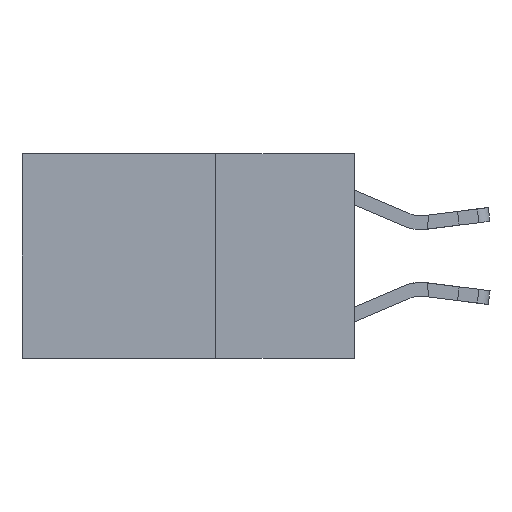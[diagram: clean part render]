
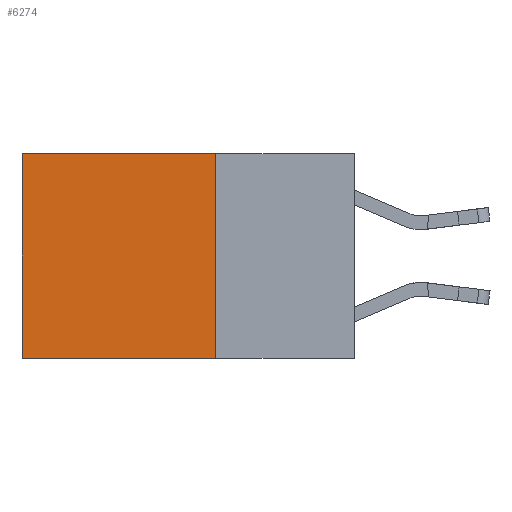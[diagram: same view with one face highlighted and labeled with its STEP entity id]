
A CAD part, left-side view. The second image highlights one B-rep face of the part: STEP entity #6274.
In plain terms, the highlighted planar face has unit normal (-1, 0, 0).
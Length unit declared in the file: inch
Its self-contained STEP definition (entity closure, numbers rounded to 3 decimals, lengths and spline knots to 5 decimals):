
#632 = DIRECTION ( 'NONE',  ( 0., 0., -1. ) ) ;
#649 = DIRECTION ( 'NONE',  ( 0., 1., 0. ) ) ;
#1404 = VECTOR ( 'NONE', #632, 39.37008 ) ;
#1470 = ORIENTED_EDGE ( 'NONE', *, *, #12815, .T. ) ;
#3358 = VERTEX_POINT ( 'NONE', #3982 ) ;
#3628 = LINE ( 'NONE', #10397, #16298 ) ;
#3683 = VECTOR ( 'NONE', #4352, 39.37008 ) ;
#3967 = DIRECTION ( 'NONE',  ( 0., 0., -1. ) ) ;
#3982 = CARTESIAN_POINT ( 'NONE',  ( 0.2625, 0.6, 0. ) ) ;
#4352 = DIRECTION ( 'NONE',  ( 0., 0., -1. ) ) ;
#4945 = LINE ( 'NONE', #13577, #6297 ) ;
#5358 = FACE_OUTER_BOUND ( 'NONE', #18333, .T. ) ;
#5976 = ORIENTED_EDGE ( 'NONE', *, *, #18044, .T. ) ;
#6274 = ADVANCED_FACE ( 'NONE', ( #5358 ), #8332, .F. ) ;
#6297 = VECTOR ( 'NONE', #15072, 39.37008 ) ;
#6619 = CARTESIAN_POINT ( 'NONE',  ( 0.2625, 0.6, -0.37 ) ) ;
#7112 = CARTESIAN_POINT ( 'NONE',  ( 0.2625, 0.25, 0. ) ) ;
#7680 = CARTESIAN_POINT ( 'NONE',  ( 0.2625, 0.6, 0. ) ) ;
#7893 = ORIENTED_EDGE ( 'NONE', *, *, #15443, .F. ) ;
#8269 = EDGE_CURVE ( 'NONE', #17693, #11674, #3628, .T. ) ;
#8332 = PLANE ( 'NONE',  #13307 ) ;
#8443 = LINE ( 'NONE', #14110, #3683 ) ;
#9579 = CARTESIAN_POINT ( 'NONE',  ( 0.2625, 0.25, -0.37 ) ) ;
#10397 = CARTESIAN_POINT ( 'NONE',  ( 0.2625, 0.25, -0.37 ) ) ;
#11674 = VERTEX_POINT ( 'NONE', #6619 ) ;
#12815 = EDGE_CURVE ( 'NONE', #15636, #3358, #4945, .T. ) ;
#13307 = AXIS2_PLACEMENT_3D ( 'NONE', #14008, #15505, #3967 ) ;
#13577 = CARTESIAN_POINT ( 'NONE',  ( 0.2625, 0.25, 0. ) ) ;
#14008 = CARTESIAN_POINT ( 'NONE',  ( 0.2625, 0.25, 0. ) ) ;
#14110 = CARTESIAN_POINT ( 'NONE',  ( 0.2625, 0.25, 0. ) ) ;
#15072 = DIRECTION ( 'NONE',  ( 0., 1., 0. ) ) ;
#15309 = ORIENTED_EDGE ( 'NONE', *, *, #8269, .F. ) ;
#15443 = EDGE_CURVE ( 'NONE', #15636, #17693, #8443, .T. ) ;
#15505 = DIRECTION ( 'NONE',  ( 1., 0., 0. ) ) ;
#15636 = VERTEX_POINT ( 'NONE', #7112 ) ;
#16154 = LINE ( 'NONE', #7680, #1404 ) ;
#16298 = VECTOR ( 'NONE', #649, 39.37008 ) ;
#17693 = VERTEX_POINT ( 'NONE', #9579 ) ;
#18044 = EDGE_CURVE ( 'NONE', #3358, #11674, #16154, .T. ) ;
#18333 = EDGE_LOOP ( 'NONE', ( #5976, #15309, #7893, #1470 ) ) ;
